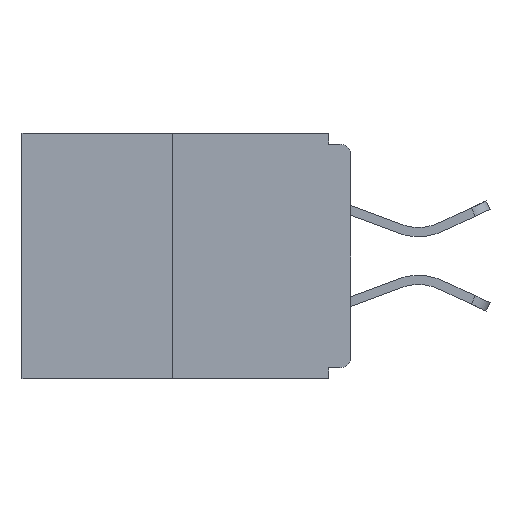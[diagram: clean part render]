
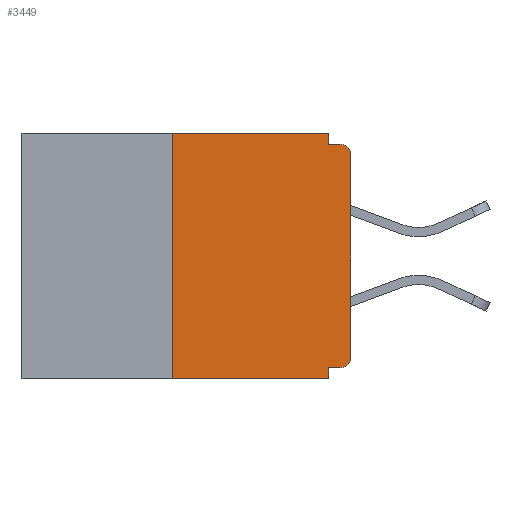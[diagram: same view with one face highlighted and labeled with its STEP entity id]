
A CAD part, left-side view. The second image highlights one B-rep face of the part: STEP entity #3449.
In plain terms, the highlighted planar face has unit normal (-1, 0, 0).
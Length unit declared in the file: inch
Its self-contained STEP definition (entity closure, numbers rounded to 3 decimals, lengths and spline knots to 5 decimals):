
#641 = ORIENTED_EDGE ( 'NONE', *, *, #13414, .F. ) ;
#701 = CIRCLE ( 'NONE', #1359, 0.015 ) ;
#858 = LINE ( 'NONE', #17256, #11364 ) ;
#909 = CARTESIAN_POINT ( 'NONE',  ( 0., 0.031, -0.343 ) ) ;
#938 = DIRECTION ( 'NONE',  ( 1., 0., 0. ) ) ;
#1180 = EDGE_CURVE ( 'NONE', #20532, #12325, #2525, .T. ) ;
#1359 = AXIS2_PLACEMENT_3D ( 'NONE', #19808, #4824, #9872 ) ;
#1794 = LINE ( 'NONE', #909, #7341 ) ;
#1815 = CIRCLE ( 'NONE', #18775, 0.015 ) ;
#2443 = LINE ( 'NONE', #10885, #19869 ) ;
#2525 = LINE ( 'NONE', #10382, #10929 ) ;
#3449 = ADVANCED_FACE ( 'NONE', ( #16443 ), #12732, .F. ) ;
#3738 = EDGE_LOOP ( 'NONE', ( #17067, #4090, #15696, #12067, #4697, #12913, #15346, #21016, #641, #21594 ) ) ;
#4029 = CARTESIAN_POINT ( 'NONE',  ( 0., 0.46, 0. ) ) ;
#4052 = VECTOR ( 'NONE', #5575, 39.37008 ) ;
#4090 = ORIENTED_EDGE ( 'NONE', *, *, #12050, .F. ) ;
#4322 = CARTESIAN_POINT ( 'NONE',  ( 0., 0.031, -0.015 ) ) ;
#4697 = ORIENTED_EDGE ( 'NONE', *, *, #17212, .F. ) ;
#4824 = DIRECTION ( 'NONE',  ( -1., 0., 0. ) ) ;
#4874 = DIRECTION ( 'NONE',  ( 0., 1., 0. ) ) ;
#5062 = AXIS2_PLACEMENT_3D ( 'NONE', #19659, #938, #19584 ) ;
#5493 = DIRECTION ( 'NONE',  ( 0., 0., 1. ) ) ;
#5575 = DIRECTION ( 'NONE',  ( 0., -1., 0. ) ) ;
#5738 = EDGE_CURVE ( 'NONE', #8176, #16587, #1815, .T. ) ;
#6129 = VERTEX_POINT ( 'NONE', #8346 ) ;
#6326 = DIRECTION ( 'NONE',  ( 0., 0., -1. ) ) ;
#6551 = EDGE_CURVE ( 'NONE', #12945, #20730, #18532, .T. ) ;
#7341 = VECTOR ( 'NONE', #7545, 39.37008 ) ;
#7545 = DIRECTION ( 'NONE',  ( 0., 0., -1. ) ) ;
#7938 = DIRECTION ( 'NONE',  ( 0., 0., 1. ) ) ;
#8176 = VERTEX_POINT ( 'NONE', #15600 ) ;
#8346 = CARTESIAN_POINT ( 'NONE',  ( 0., 0., -0.03 ) ) ;
#8916 = EDGE_CURVE ( 'NONE', #9417, #12325, #1794, .T. ) ;
#9417 = VERTEX_POINT ( 'NONE', #18406 ) ;
#9872 = DIRECTION ( 'NONE',  ( 0., 0., -1. ) ) ;
#10008 = CARTESIAN_POINT ( 'NONE',  ( 0., 0., -0.328 ) ) ;
#10382 = CARTESIAN_POINT ( 'NONE',  ( 0., 0.46, -0.343 ) ) ;
#10885 = CARTESIAN_POINT ( 'NONE',  ( 0., 0., -0.015 ) ) ;
#10929 = VECTOR ( 'NONE', #13663, 39.37008 ) ;
#11137 = VERTEX_POINT ( 'NONE', #21612 ) ;
#11310 = DIRECTION ( 'NONE',  ( -1., 0., 0. ) ) ;
#11364 = VECTOR ( 'NONE', #5493, 39.37008 ) ;
#12050 = EDGE_CURVE ( 'NONE', #20532, #11137, #12203, .T. ) ;
#12067 = ORIENTED_EDGE ( 'NONE', *, *, #8916, .F. ) ;
#12203 = LINE ( 'NONE', #19752, #21759 ) ;
#12284 = EDGE_CURVE ( 'NONE', #16587, #6129, #858, .T. ) ;
#12325 = VERTEX_POINT ( 'NONE', #15544 ) ;
#12732 = PLANE ( 'NONE',  #5062 ) ;
#12913 = ORIENTED_EDGE ( 'NONE', *, *, #5738, .T. ) ;
#12945 = VERTEX_POINT ( 'NONE', #13823 ) ;
#13074 = CARTESIAN_POINT ( 'NONE',  ( 0., 0.031, 0. ) ) ;
#13414 = EDGE_CURVE ( 'NONE', #20730, #14391, #2443, .T. ) ;
#13663 = DIRECTION ( 'NONE',  ( 0., -1., 0. ) ) ;
#13823 = CARTESIAN_POINT ( 'NONE',  ( 0., 0.031, 0. ) ) ;
#14360 = CARTESIAN_POINT ( 'NONE',  ( 0., 0.015, -0.015 ) ) ;
#14391 = VERTEX_POINT ( 'NONE', #14360 ) ;
#14662 = VECTOR ( 'NONE', #4874, 39.37008 ) ;
#15198 = LINE ( 'NONE', #10008, #14662 ) ;
#15346 = ORIENTED_EDGE ( 'NONE', *, *, #12284, .T. ) ;
#15544 = CARTESIAN_POINT ( 'NONE',  ( 0., 0.031, -0.343 ) ) ;
#15600 = CARTESIAN_POINT ( 'NONE',  ( 0., 0.015, -0.328 ) ) ;
#15696 = ORIENTED_EDGE ( 'NONE', *, *, #1180, .T. ) ;
#16443 = FACE_OUTER_BOUND ( 'NONE', #3738, .T. ) ;
#16587 = VERTEX_POINT ( 'NONE', #20033 ) ;
#16657 = EDGE_CURVE ( 'NONE', #6129, #14391, #701, .T. ) ;
#17067 = ORIENTED_EDGE ( 'NONE', *, *, #18178, .F. ) ;
#17212 = EDGE_CURVE ( 'NONE', #8176, #9417, #15198, .T. ) ;
#17256 = CARTESIAN_POINT ( 'NONE',  ( 0., 0., 0. ) ) ;
#17743 = DIRECTION ( 'NONE',  ( 0., -1., 0. ) ) ;
#18178 = EDGE_CURVE ( 'NONE', #11137, #12945, #19365, .T. ) ;
#18184 = DIRECTION ( 'NONE',  ( 0., 0., -1. ) ) ;
#18406 = CARTESIAN_POINT ( 'NONE',  ( 0., 0.031, -0.328 ) ) ;
#18532 = LINE ( 'NONE', #13074, #19826 ) ;
#18775 = AXIS2_PLACEMENT_3D ( 'NONE', #21582, #11310, #6326 ) ;
#19365 = LINE ( 'NONE', #4029, #4052 ) ;
#19584 = DIRECTION ( 'NONE',  ( 0., 0., -1. ) ) ;
#19659 = CARTESIAN_POINT ( 'NONE',  ( 0., 0.46, 0. ) ) ;
#19752 = CARTESIAN_POINT ( 'NONE',  ( 0., 0.25, 0. ) ) ;
#19808 = CARTESIAN_POINT ( 'NONE',  ( 0., 0.015, -0.03 ) ) ;
#19826 = VECTOR ( 'NONE', #18184, 39.37008 ) ;
#19869 = VECTOR ( 'NONE', #17743, 39.37008 ) ;
#20033 = CARTESIAN_POINT ( 'NONE',  ( 0., 0., -0.313 ) ) ;
#20532 = VERTEX_POINT ( 'NONE', #21106 ) ;
#20730 = VERTEX_POINT ( 'NONE', #4322 ) ;
#21016 = ORIENTED_EDGE ( 'NONE', *, *, #16657, .T. ) ;
#21106 = CARTESIAN_POINT ( 'NONE',  ( 0., 0.25, -0.343 ) ) ;
#21582 = CARTESIAN_POINT ( 'NONE',  ( 0., 0.015, -0.313 ) ) ;
#21594 = ORIENTED_EDGE ( 'NONE', *, *, #6551, .F. ) ;
#21612 = CARTESIAN_POINT ( 'NONE',  ( 0., 0.25, 0. ) ) ;
#21759 = VECTOR ( 'NONE', #7938, 39.37008 ) ;
